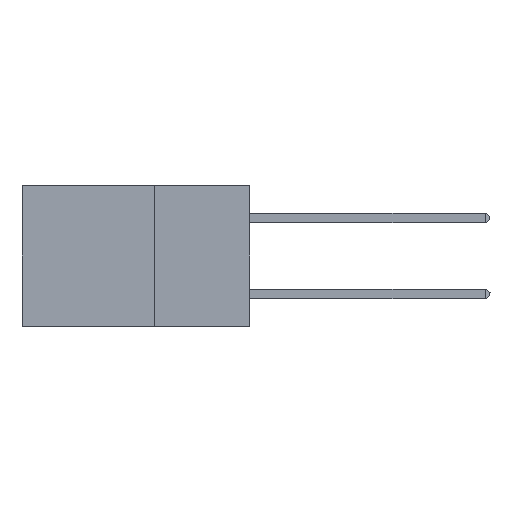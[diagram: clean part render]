
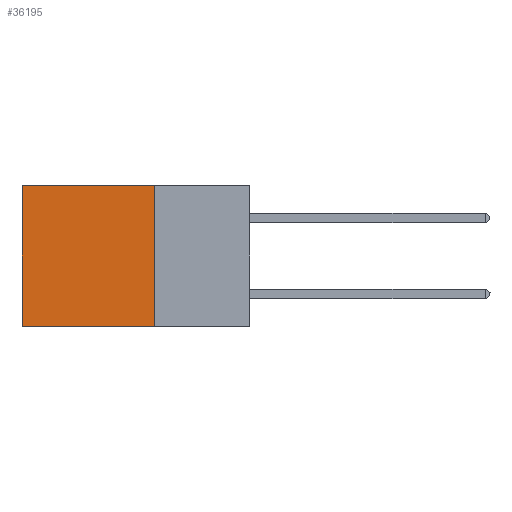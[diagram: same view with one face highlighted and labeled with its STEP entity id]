
A CAD part, left-side view. The second image highlights one B-rep face of the part: STEP entity #36195.
In plain terms, the highlighted planar face has unit normal (-1, 0, 0).
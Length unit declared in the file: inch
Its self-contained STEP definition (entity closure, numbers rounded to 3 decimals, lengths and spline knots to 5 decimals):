
#1291 = CARTESIAN_POINT ( 'NONE',  ( 0.2875, 0.25, 0. ) ) ;
#2636 = CARTESIAN_POINT ( 'NONE',  ( 0.2875, 0.25, -0.37 ) ) ;
#5318 = PLANE ( 'NONE',  #34577 ) ;
#5889 = DIRECTION ( 'NONE',  ( 0., 0., -1. ) ) ;
#7758 = CARTESIAN_POINT ( 'NONE',  ( 0.2875, 0.25, 0. ) ) ;
#8235 = EDGE_CURVE ( 'NONE', #37689, #22558, #36470, .T. ) ;
#8913 = CARTESIAN_POINT ( 'NONE',  ( 0.2875, 0.6, 0. ) ) ;
#11291 = LINE ( 'NONE', #1291, #30279 ) ;
#12580 = EDGE_CURVE ( 'NONE', #16324, #22959, #11291, .T. ) ;
#13464 = ORIENTED_EDGE ( 'NONE', *, *, #35860, .T. ) ;
#13651 = DIRECTION ( 'NONE',  ( 0., 1., 0. ) ) ;
#16324 = VERTEX_POINT ( 'NONE', #30119 ) ;
#18290 = ORIENTED_EDGE ( 'NONE', *, *, #27271, .F. ) ;
#20406 = CARTESIAN_POINT ( 'NONE',  ( 0.2875, 0.25, -0.37 ) ) ;
#22558 = VERTEX_POINT ( 'NONE', #28396 ) ;
#22959 = VERTEX_POINT ( 'NONE', #20406 ) ;
#25308 = CARTESIAN_POINT ( 'NONE',  ( 0.2875, 0.25, 0. ) ) ;
#25528 = ORIENTED_EDGE ( 'NONE', *, *, #8235, .T. ) ;
#25692 = DIRECTION ( 'NONE',  ( 0., 0., -1. ) ) ;
#26517 = ORIENTED_EDGE ( 'NONE', *, *, #12580, .F. ) ;
#27271 = EDGE_CURVE ( 'NONE', #22959, #22558, #29833, .T. ) ;
#28396 = CARTESIAN_POINT ( 'NONE',  ( 0.2875, 0.6, -0.37 ) ) ;
#28608 = DIRECTION ( 'NONE',  ( 1., 0., 0. ) ) ;
#28648 = DIRECTION ( 'NONE',  ( 0., 0., -1. ) ) ;
#29431 = VECTOR ( 'NONE', #13651, 39.37008 ) ;
#29833 = LINE ( 'NONE', #2636, #37053 ) ;
#30119 = CARTESIAN_POINT ( 'NONE',  ( 0.2875, 0.25, 0. ) ) ;
#30279 = VECTOR ( 'NONE', #28648, 39.37008 ) ;
#33401 = VECTOR ( 'NONE', #25692, 39.37008 ) ;
#34577 = AXIS2_PLACEMENT_3D ( 'NONE', #25308, #28608, #5889 ) ;
#34584 = FACE_OUTER_BOUND ( 'NONE', #41321, .T. ) ;
#35860 = EDGE_CURVE ( 'NONE', #16324, #37689, #36587, .T. ) ;
#36195 = ADVANCED_FACE ( 'NONE', ( #34584 ), #5318, .F. ) ;
#36470 = LINE ( 'NONE', #38727, #33401 ) ;
#36587 = LINE ( 'NONE', #7758, #29431 ) ;
#37053 = VECTOR ( 'NONE', #38963, 39.37008 ) ;
#37689 = VERTEX_POINT ( 'NONE', #8913 ) ;
#38727 = CARTESIAN_POINT ( 'NONE',  ( 0.2875, 0.6, 0. ) ) ;
#38963 = DIRECTION ( 'NONE',  ( 0., 1., 0. ) ) ;
#41321 = EDGE_LOOP ( 'NONE', ( #25528, #18290, #26517, #13464 ) ) ;
